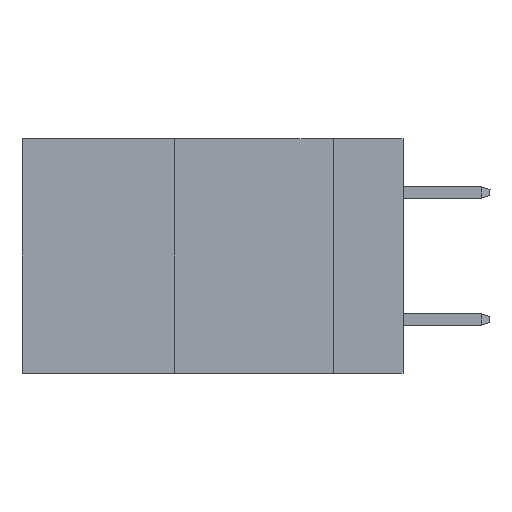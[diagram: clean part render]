
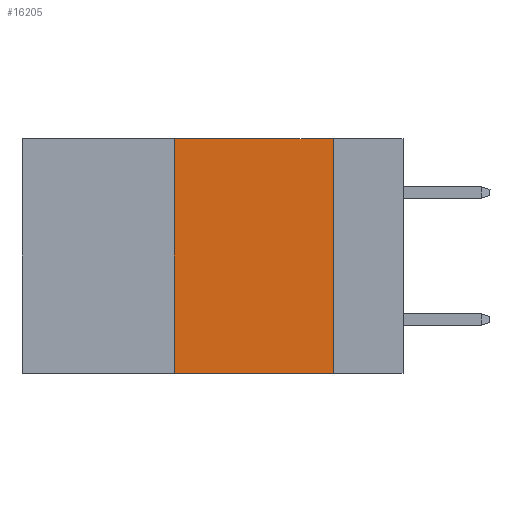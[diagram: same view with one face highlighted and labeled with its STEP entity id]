
A CAD part, left-side view. The second image highlights one B-rep face of the part: STEP entity #16205.
In plain terms, the highlighted planar face has unit normal (-1, 0, 0).
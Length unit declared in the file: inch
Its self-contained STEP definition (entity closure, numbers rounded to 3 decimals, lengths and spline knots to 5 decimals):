
#745 = CARTESIAN_POINT ( 'NONE',  ( 0., 0.36, 0. ) ) ;
#866 = CARTESIAN_POINT ( 'NONE',  ( 0., 0.6, 0. ) ) ;
#1147 = LINE ( 'NONE', #7335, #7220 ) ;
#1469 = FACE_OUTER_BOUND ( 'NONE', #2400, .T. ) ;
#1548 = ORIENTED_EDGE ( 'NONE', *, *, #3604, .F. ) ;
#1647 = CARTESIAN_POINT ( 'NONE',  ( 0., 0.36, -0.37 ) ) ;
#1876 = AXIS2_PLACEMENT_3D ( 'NONE', #13196, #12866, #10207 ) ;
#1893 = VERTEX_POINT ( 'NONE', #1647 ) ;
#2400 = EDGE_LOOP ( 'NONE', ( #15063, #1548, #13603, #3252 ) ) ;
#3216 = VECTOR ( 'NONE', #3226, 39.37008 ) ;
#3226 = DIRECTION ( 'NONE',  ( 0., -1., 0. ) ) ;
#3252 = ORIENTED_EDGE ( 'NONE', *, *, #5066, .T. ) ;
#3477 = LINE ( 'NONE', #866, #3216 ) ;
#3604 = EDGE_CURVE ( 'NONE', #15978, #13766, #3477, .T. ) ;
#4817 = VECTOR ( 'NONE', #10054, 39.37008 ) ;
#5066 = EDGE_CURVE ( 'NONE', #1893, #9195, #5222, .T. ) ;
#5222 = LINE ( 'NONE', #11944, #8222 ) ;
#6001 = DIRECTION ( 'NONE',  ( 0., 0., -1. ) ) ;
#6657 = PLANE ( 'NONE',  #1876 ) ;
#7220 = VECTOR ( 'NONE', #6001, 39.37008 ) ;
#7335 = CARTESIAN_POINT ( 'NONE',  ( 0., 0.11, 0. ) ) ;
#8222 = VECTOR ( 'NONE', #9276, 39.37008 ) ;
#8763 = LINE ( 'NONE', #11510, #4817 ) ;
#9195 = VERTEX_POINT ( 'NONE', #10482 ) ;
#9276 = DIRECTION ( 'NONE',  ( 0., -1., 0. ) ) ;
#10054 = DIRECTION ( 'NONE',  ( 0., 0., 1. ) ) ;
#10207 = DIRECTION ( 'NONE',  ( 0., 0., -1. ) ) ;
#10482 = CARTESIAN_POINT ( 'NONE',  ( 0., 0.11, -0.37 ) ) ;
#11510 = CARTESIAN_POINT ( 'NONE',  ( 0., 0.36, 0. ) ) ;
#11944 = CARTESIAN_POINT ( 'NONE',  ( 0., 0.6, -0.37 ) ) ;
#12124 = CARTESIAN_POINT ( 'NONE',  ( 0., 0.11, 0. ) ) ;
#12536 = EDGE_CURVE ( 'NONE', #1893, #15978, #8763, .T. ) ;
#12866 = DIRECTION ( 'NONE',  ( 1., 0., 0. ) ) ;
#13196 = CARTESIAN_POINT ( 'NONE',  ( 0., 0.6, 0. ) ) ;
#13603 = ORIENTED_EDGE ( 'NONE', *, *, #12536, .F. ) ;
#13766 = VERTEX_POINT ( 'NONE', #12124 ) ;
#14187 = EDGE_CURVE ( 'NONE', #13766, #9195, #1147, .T. ) ;
#15063 = ORIENTED_EDGE ( 'NONE', *, *, #14187, .F. ) ;
#15978 = VERTEX_POINT ( 'NONE', #745 ) ;
#16205 = ADVANCED_FACE ( 'NONE', ( #1469 ), #6657, .F. ) ;
